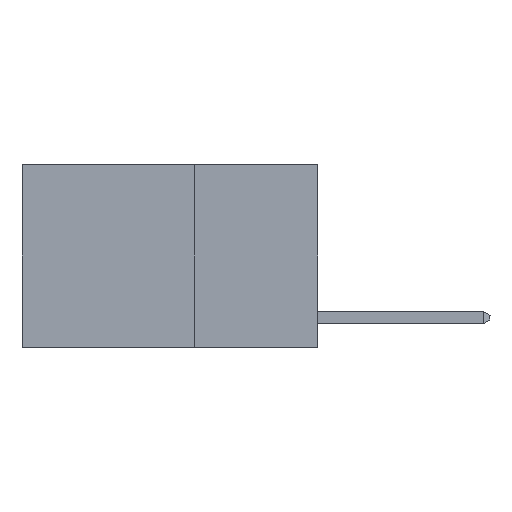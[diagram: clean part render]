
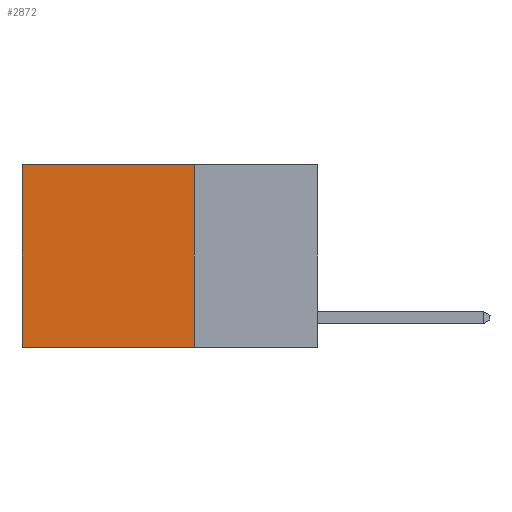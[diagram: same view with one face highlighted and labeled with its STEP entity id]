
A CAD part, left-side view. The second image highlights one B-rep face of the part: STEP entity #2872.
In plain terms, the highlighted planar face has unit normal (-1, 0, 0).
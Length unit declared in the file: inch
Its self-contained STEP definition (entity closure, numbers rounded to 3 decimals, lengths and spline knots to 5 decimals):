
#159 = EDGE_CURVE ( 'NONE', #2791, #6289, #9037, .T. ) ;
#489 = VERTEX_POINT ( 'NONE', #3217 ) ;
#984 = LINE ( 'NONE', #12860, #9254 ) ;
#1003 = ORIENTED_EDGE ( 'NONE', *, *, #159, .F. ) ;
#1025 = DIRECTION ( 'NONE',  ( 0., 1., 0. ) ) ;
#1037 = EDGE_CURVE ( 'NONE', #7457, #489, #10440, .T. ) ;
#1069 = ORIENTED_EDGE ( 'NONE', *, *, #2984, .T. ) ;
#1517 = DIRECTION ( 'NONE',  ( 0., 0., -1. ) ) ;
#1570 = PLANE ( 'NONE',  #8219 ) ;
#2791 = VERTEX_POINT ( 'NONE', #11464 ) ;
#2872 = ADVANCED_FACE ( 'NONE', ( #4590 ), #1570, .F. ) ;
#2984 = EDGE_CURVE ( 'NONE', #2791, #7457, #984, .T. ) ;
#3053 = CARTESIAN_POINT ( 'NONE',  ( 0.2625, 0.25, -0.37 ) ) ;
#3112 = CARTESIAN_POINT ( 'NONE',  ( 0.2625, 0.25, 0. ) ) ;
#3217 = CARTESIAN_POINT ( 'NONE',  ( 0.2625, 0.6, -0.37 ) ) ;
#4590 = FACE_OUTER_BOUND ( 'NONE', #7578, .T. ) ;
#5364 = EDGE_CURVE ( 'NONE', #6289, #489, #8928, .T. ) ;
#5549 = DIRECTION ( 'NONE',  ( 0., 0., -1. ) ) ;
#5880 = CARTESIAN_POINT ( 'NONE',  ( 0.2625, 0.25, -0.37 ) ) ;
#6257 = VECTOR ( 'NONE', #7087, 39.37008 ) ;
#6289 = VERTEX_POINT ( 'NONE', #5880 ) ;
#6851 = DIRECTION ( 'NONE',  ( 0., 1., 0. ) ) ;
#7087 = DIRECTION ( 'NONE',  ( 0., 0., -1. ) ) ;
#7457 = VERTEX_POINT ( 'NONE', #9684 ) ;
#7578 = EDGE_LOOP ( 'NONE', ( #12556, #10266, #1003, #1069 ) ) ;
#8219 = AXIS2_PLACEMENT_3D ( 'NONE', #12733, #9726, #5549 ) ;
#8928 = LINE ( 'NONE', #3053, #11738 ) ;
#9037 = LINE ( 'NONE', #3112, #6257 ) ;
#9254 = VECTOR ( 'NONE', #6851, 39.37008 ) ;
#9684 = CARTESIAN_POINT ( 'NONE',  ( 0.2625, 0.6, 0. ) ) ;
#9726 = DIRECTION ( 'NONE',  ( 1., 0., 0. ) ) ;
#10266 = ORIENTED_EDGE ( 'NONE', *, *, #5364, .F. ) ;
#10440 = LINE ( 'NONE', #12350, #12112 ) ;
#11464 = CARTESIAN_POINT ( 'NONE',  ( 0.2625, 0.25, 0. ) ) ;
#11738 = VECTOR ( 'NONE', #1025, 39.37008 ) ;
#12112 = VECTOR ( 'NONE', #1517, 39.37008 ) ;
#12350 = CARTESIAN_POINT ( 'NONE',  ( 0.2625, 0.6, 0. ) ) ;
#12556 = ORIENTED_EDGE ( 'NONE', *, *, #1037, .T. ) ;
#12733 = CARTESIAN_POINT ( 'NONE',  ( 0.2625, 0.25, 0. ) ) ;
#12860 = CARTESIAN_POINT ( 'NONE',  ( 0.2625, 0.25, 0. ) ) ;
